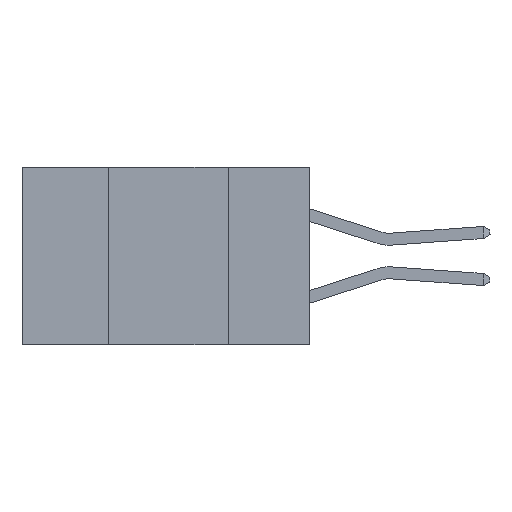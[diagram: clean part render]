
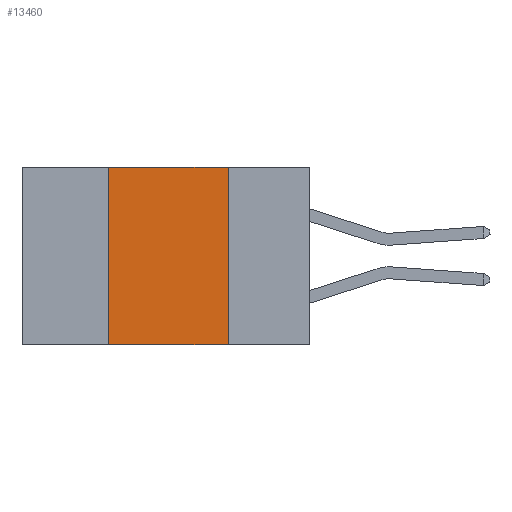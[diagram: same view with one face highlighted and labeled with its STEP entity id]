
A CAD part, left-side view. The second image highlights one B-rep face of the part: STEP entity #13460.
In plain terms, the highlighted planar face has unit normal (-1, 0, 0).
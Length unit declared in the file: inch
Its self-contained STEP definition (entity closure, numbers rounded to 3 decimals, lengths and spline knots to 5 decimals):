
#261 = CARTESIAN_POINT ( 'NONE',  ( 0., 0.6, 0. ) ) ;
#1353 = CARTESIAN_POINT ( 'NONE',  ( 0., 0.42, 0. ) ) ;
#1395 = EDGE_CURVE ( 'NONE', #9784, #4227, #19265, .T. ) ;
#1831 = DIRECTION ( 'NONE',  ( 0., 0., -1. ) ) ;
#4007 = AXIS2_PLACEMENT_3D ( 'NONE', #261, #11055, #1831 ) ;
#4227 = VERTEX_POINT ( 'NONE', #6906 ) ;
#4300 = LINE ( 'NONE', #17753, #11990 ) ;
#4509 = FACE_OUTER_BOUND ( 'NONE', #8509, .T. ) ;
#4523 = CARTESIAN_POINT ( 'NONE',  ( 0., 0.6, 0. ) ) ;
#5599 = DIRECTION ( 'NONE',  ( 0., 0., 1. ) ) ;
#6549 = EDGE_CURVE ( 'NONE', #9784, #9286, #14962, .T. ) ;
#6648 = VERTEX_POINT ( 'NONE', #12177 ) ;
#6906 = CARTESIAN_POINT ( 'NONE',  ( 0., 0.17, -0.37 ) ) ;
#7627 = VECTOR ( 'NONE', #5599, 39.37008 ) ;
#8509 = EDGE_LOOP ( 'NONE', ( #8861, #9672, #14774, #13627 ) ) ;
#8861 = ORIENTED_EDGE ( 'NONE', *, *, #12773, .F. ) ;
#9286 = VERTEX_POINT ( 'NONE', #1353 ) ;
#9539 = LINE ( 'NONE', #4523, #17250 ) ;
#9672 = ORIENTED_EDGE ( 'NONE', *, *, #11575, .F. ) ;
#9784 = VERTEX_POINT ( 'NONE', #11076 ) ;
#11055 = DIRECTION ( 'NONE',  ( 1., 0., 0. ) ) ;
#11076 = CARTESIAN_POINT ( 'NONE',  ( 0., 0.42, -0.37 ) ) ;
#11225 = VECTOR ( 'NONE', #18323, 39.37008 ) ;
#11575 = EDGE_CURVE ( 'NONE', #9286, #6648, #9539, .T. ) ;
#11990 = VECTOR ( 'NONE', #15527, 39.37008 ) ;
#12177 = CARTESIAN_POINT ( 'NONE',  ( 0., 0.17, 0. ) ) ;
#12773 = EDGE_CURVE ( 'NONE', #6648, #4227, #4300, .T. ) ;
#13460 = ADVANCED_FACE ( 'NONE', ( #4509 ), #15651, .F. ) ;
#13627 = ORIENTED_EDGE ( 'NONE', *, *, #1395, .T. ) ;
#14774 = ORIENTED_EDGE ( 'NONE', *, *, #6549, .F. ) ;
#14822 = CARTESIAN_POINT ( 'NONE',  ( 0., 0.42, 0. ) ) ;
#14962 = LINE ( 'NONE', #14822, #7627 ) ;
#15292 = DIRECTION ( 'NONE',  ( 0., -1., 0. ) ) ;
#15527 = DIRECTION ( 'NONE',  ( 0., 0., -1. ) ) ;
#15651 = PLANE ( 'NONE',  #4007 ) ;
#17250 = VECTOR ( 'NONE', #15292, 39.37008 ) ;
#17753 = CARTESIAN_POINT ( 'NONE',  ( 0., 0.17, 0. ) ) ;
#18323 = DIRECTION ( 'NONE',  ( 0., -1., 0. ) ) ;
#18879 = CARTESIAN_POINT ( 'NONE',  ( 0., 0.6, -0.37 ) ) ;
#19265 = LINE ( 'NONE', #18879, #11225 ) ;
